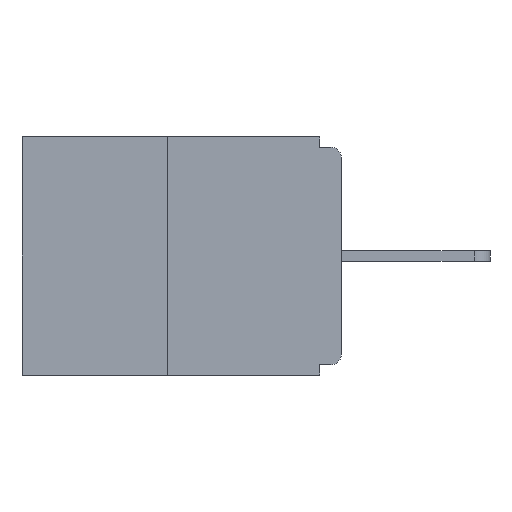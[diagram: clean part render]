
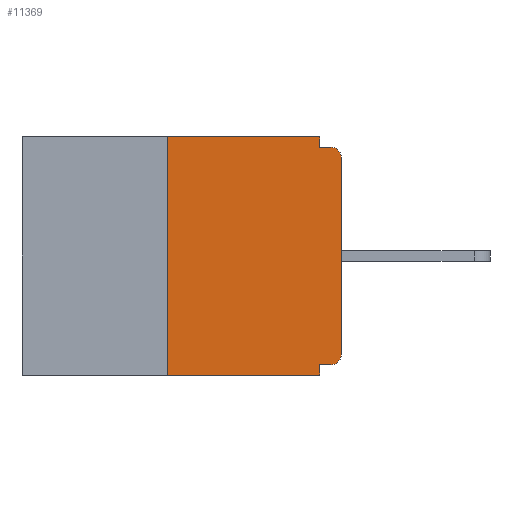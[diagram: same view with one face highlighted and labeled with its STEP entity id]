
A CAD part, left-side view. The second image highlights one B-rep face of the part: STEP entity #11369.
In plain terms, the highlighted planar face has unit normal (-1, 0, 0).
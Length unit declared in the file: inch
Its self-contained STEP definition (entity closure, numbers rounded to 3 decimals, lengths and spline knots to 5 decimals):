
#57 = VERTEX_POINT ( 'NONE', #388 ) ;
#136 = CARTESIAN_POINT ( 'NONE',  ( 0., 0.46, 0. ) ) ;
#305 = VECTOR ( 'NONE', #4188, 39.37008 ) ;
#388 = CARTESIAN_POINT ( 'NONE',  ( 0., 0.25, 0. ) ) ;
#862 = CIRCLE ( 'NONE', #10514, 0.015 ) ;
#1097 = VECTOR ( 'NONE', #13438, 39.37008 ) ;
#1357 = ORIENTED_EDGE ( 'NONE', *, *, #17083, .F. ) ;
#1526 = DIRECTION ( 'NONE',  ( 1., 0., 0. ) ) ;
#1820 = CARTESIAN_POINT ( 'NONE',  ( 0., 0.031, -0.015 ) ) ;
#1983 = VECTOR ( 'NONE', #14347, 39.37008 ) ;
#2220 = CARTESIAN_POINT ( 'NONE',  ( 0., 0.015, -0.328 ) ) ;
#2545 = CARTESIAN_POINT ( 'NONE',  ( 0., 0., -0.03 ) ) ;
#2733 = CIRCLE ( 'NONE', #4222, 0.015 ) ;
#3026 = VERTEX_POINT ( 'NONE', #16139 ) ;
#3445 = CARTESIAN_POINT ( 'NONE',  ( 0., 0.25, -0.343 ) ) ;
#3976 = LINE ( 'NONE', #16227, #305 ) ;
#4085 = EDGE_CURVE ( 'NONE', #11632, #57, #16612, .T. ) ;
#4093 = CARTESIAN_POINT ( 'NONE',  ( 0., 0., -0.328 ) ) ;
#4188 = DIRECTION ( 'NONE',  ( 0., -1., 0. ) ) ;
#4205 = VERTEX_POINT ( 'NONE', #2220 ) ;
#4222 = AXIS2_PLACEMENT_3D ( 'NONE', #15024, #6945, #16323 ) ;
#4409 = VERTEX_POINT ( 'NONE', #16907 ) ;
#4626 = LINE ( 'NONE', #4093, #14977 ) ;
#4727 = LINE ( 'NONE', #14435, #15082 ) ;
#4985 = DIRECTION ( 'NONE',  ( 0., 0., -1. ) ) ;
#5125 = DIRECTION ( 'NONE',  ( 0., 0., 1. ) ) ;
#5347 = LINE ( 'NONE', #5373, #8539 ) ;
#5373 = CARTESIAN_POINT ( 'NONE',  ( 0., 0., 0. ) ) ;
#5453 = CARTESIAN_POINT ( 'NONE',  ( 0., 0.25, 0. ) ) ;
#5815 = CARTESIAN_POINT ( 'NONE',  ( 0., 0.015, -0.313 ) ) ;
#6236 = ORIENTED_EDGE ( 'NONE', *, *, #4085, .F. ) ;
#6938 = AXIS2_PLACEMENT_3D ( 'NONE', #136, #1526, #11067 ) ;
#6945 = DIRECTION ( 'NONE',  ( -1., 0., 0. ) ) ;
#7198 = DIRECTION ( 'NONE',  ( 0., 0., -1. ) ) ;
#7478 = EDGE_CURVE ( 'NONE', #10827, #8657, #5347, .T. ) ;
#7983 = ORIENTED_EDGE ( 'NONE', *, *, #11364, .T. ) ;
#7998 = ORIENTED_EDGE ( 'NONE', *, *, #16872, .T. ) ;
#8324 = PLANE ( 'NONE',  #6938 ) ;
#8539 = VECTOR ( 'NONE', #12568, 39.37008 ) ;
#8579 = VECTOR ( 'NONE', #10802, 39.37008 ) ;
#8657 = VERTEX_POINT ( 'NONE', #2545 ) ;
#8991 = LINE ( 'NONE', #9419, #8579 ) ;
#9204 = LINE ( 'NONE', #13043, #1983 ) ;
#9419 = CARTESIAN_POINT ( 'NONE',  ( 0., 0.46, -0.343 ) ) ;
#10342 = VERTEX_POINT ( 'NONE', #15749 ) ;
#10514 = AXIS2_PLACEMENT_3D ( 'NONE', #5815, #15260, #7198 ) ;
#10802 = DIRECTION ( 'NONE',  ( 0., -1., 0. ) ) ;
#10827 = VERTEX_POINT ( 'NONE', #12834 ) ;
#11067 = DIRECTION ( 'NONE',  ( 0., 0., -1. ) ) ;
#11364 = EDGE_CURVE ( 'NONE', #8657, #10342, #2733, .T. ) ;
#11369 = ADVANCED_FACE ( 'NONE', ( #13572 ), #8324, .F. ) ;
#11380 = ORIENTED_EDGE ( 'NONE', *, *, #13789, .F. ) ;
#11506 = VERTEX_POINT ( 'NONE', #1820 ) ;
#11632 = VERTEX_POINT ( 'NONE', #3445 ) ;
#11816 = VERTEX_POINT ( 'NONE', #12000 ) ;
#11914 = EDGE_CURVE ( 'NONE', #4205, #4409, #4626, .T. ) ;
#11997 = LINE ( 'NONE', #12098, #1097 ) ;
#12000 = CARTESIAN_POINT ( 'NONE',  ( 0., 0.031, -0.343 ) ) ;
#12098 = CARTESIAN_POINT ( 'NONE',  ( 0., 0.031, -0.343 ) ) ;
#12568 = DIRECTION ( 'NONE',  ( 0., 0., 1. ) ) ;
#12578 = EDGE_CURVE ( 'NONE', #11506, #10342, #3976, .T. ) ;
#12834 = CARTESIAN_POINT ( 'NONE',  ( 0., 0., -0.313 ) ) ;
#13043 = CARTESIAN_POINT ( 'NONE',  ( 0., 0.46, 0. ) ) ;
#13082 = ORIENTED_EDGE ( 'NONE', *, *, #12578, .F. ) ;
#13114 = EDGE_LOOP ( 'NONE', ( #11380, #6236, #15793, #15282, #16739, #7998, #17350, #7983, #13082, #1357 ) ) ;
#13142 = VECTOR ( 'NONE', #5125, 39.37008 ) ;
#13438 = DIRECTION ( 'NONE',  ( 0., 0., -1. ) ) ;
#13572 = FACE_OUTER_BOUND ( 'NONE', #13114, .T. ) ;
#13619 = EDGE_CURVE ( 'NONE', #11632, #11816, #8991, .T. ) ;
#13789 = EDGE_CURVE ( 'NONE', #57, #3026, #9204, .T. ) ;
#14347 = DIRECTION ( 'NONE',  ( 0., -1., 0. ) ) ;
#14435 = CARTESIAN_POINT ( 'NONE',  ( 0., 0.031, 0. ) ) ;
#14884 = DIRECTION ( 'NONE',  ( 0., 1., 0. ) ) ;
#14977 = VECTOR ( 'NONE', #14884, 39.37008 ) ;
#15024 = CARTESIAN_POINT ( 'NONE',  ( 0., 0.015, -0.03 ) ) ;
#15082 = VECTOR ( 'NONE', #4985, 39.37008 ) ;
#15260 = DIRECTION ( 'NONE',  ( -1., 0., 0. ) ) ;
#15282 = ORIENTED_EDGE ( 'NONE', *, *, #16641, .F. ) ;
#15749 = CARTESIAN_POINT ( 'NONE',  ( 0., 0.015, -0.015 ) ) ;
#15793 = ORIENTED_EDGE ( 'NONE', *, *, #13619, .T. ) ;
#16139 = CARTESIAN_POINT ( 'NONE',  ( 0., 0.031, 0. ) ) ;
#16227 = CARTESIAN_POINT ( 'NONE',  ( 0., 0., -0.015 ) ) ;
#16323 = DIRECTION ( 'NONE',  ( 0., 0., -1. ) ) ;
#16612 = LINE ( 'NONE', #5453, #13142 ) ;
#16641 = EDGE_CURVE ( 'NONE', #4409, #11816, #11997, .T. ) ;
#16739 = ORIENTED_EDGE ( 'NONE', *, *, #11914, .F. ) ;
#16872 = EDGE_CURVE ( 'NONE', #4205, #10827, #862, .T. ) ;
#16907 = CARTESIAN_POINT ( 'NONE',  ( 0., 0.031, -0.328 ) ) ;
#17083 = EDGE_CURVE ( 'NONE', #3026, #11506, #4727, .T. ) ;
#17350 = ORIENTED_EDGE ( 'NONE', *, *, #7478, .T. ) ;
